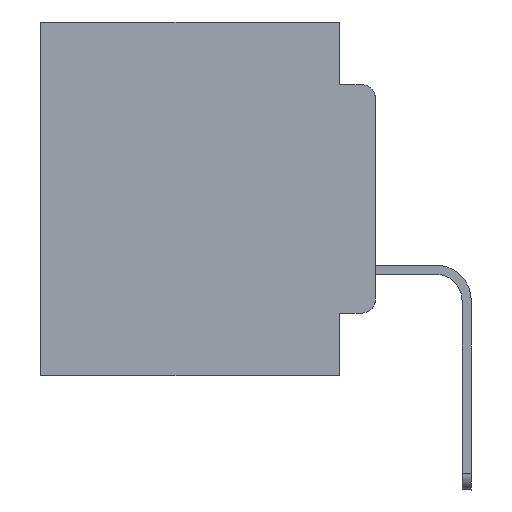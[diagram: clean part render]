
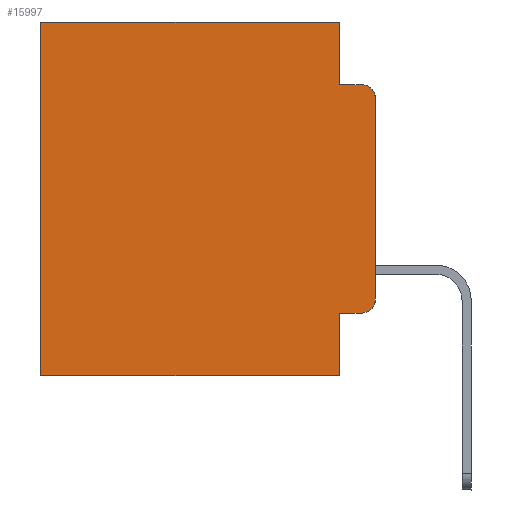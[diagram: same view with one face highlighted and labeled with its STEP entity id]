
A CAD part, left-side view. The second image highlights one B-rep face of the part: STEP entity #15997.
In plain terms, the highlighted planar face has unit normal (-1, 0, 0).
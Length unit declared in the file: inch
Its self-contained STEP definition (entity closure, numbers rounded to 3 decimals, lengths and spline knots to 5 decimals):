
#110 = LINE ( 'NONE', #13488, #19756 ) ;
#147 = DIRECTION ( 'NONE',  ( -1., 0., 0. ) ) ;
#587 = ORIENTED_EDGE ( 'NONE', *, *, #12937, .T. ) ;
#695 = ORIENTED_EDGE ( 'NONE', *, *, #14527, .F. ) ;
#725 = ORIENTED_EDGE ( 'NONE', *, *, #23851, .T. ) ;
#1013 = VERTEX_POINT ( 'NONE', #10838 ) ;
#1475 = LINE ( 'NONE', #11802, #9394 ) ;
#1532 = AXIS2_PLACEMENT_3D ( 'NONE', #22654, #147, #18712 ) ;
#1558 = CARTESIAN_POINT ( 'NONE',  ( 0.298, 0.02, -0.0885 ) ) ;
#2122 = EDGE_CURVE ( 'NONE', #12835, #20879, #1475, .T. ) ;
#2911 = VECTOR ( 'NONE', #20334, 39.37008 ) ;
#2927 = LINE ( 'NONE', #21885, #21627 ) ;
#3465 = CARTESIAN_POINT ( 'NONE',  ( 0.298, 0.051, 0. ) ) ;
#4280 = EDGE_CURVE ( 'NONE', #16893, #9608, #2927, .T. ) ;
#4415 = VECTOR ( 'NONE', #14277, 39.37008 ) ;
#4571 = CARTESIAN_POINT ( 'NONE',  ( 0.298, 0.051, 0. ) ) ;
#4652 = DIRECTION ( 'NONE',  ( 0., 0., -1. ) ) ;
#5561 = CARTESIAN_POINT ( 'NONE',  ( 0.298, 0.02, -0.1085 ) ) ;
#5987 = CARTESIAN_POINT ( 'NONE',  ( 0.298, 0.051, -0.0885 ) ) ;
#6456 = VERTEX_POINT ( 'NONE', #5987 ) ;
#7241 = EDGE_CURVE ( 'NONE', #9608, #1013, #21271, .T. ) ;
#7259 = ORIENTED_EDGE ( 'NONE', *, *, #4280, .F. ) ;
#7428 = DIRECTION ( 'NONE',  ( 0., 0., -1. ) ) ;
#7783 = ORIENTED_EDGE ( 'NONE', *, *, #13882, .T. ) ;
#7812 = DIRECTION ( 'NONE',  ( 0., -1., 0. ) ) ;
#8128 = PLANE ( 'NONE',  #25142 ) ;
#8304 = DIRECTION ( 'NONE',  ( 0., 0., -1. ) ) ;
#8321 = CIRCLE ( 'NONE', #24081, 0.02 ) ;
#9292 = EDGE_CURVE ( 'NONE', #9637, #18678, #14882, .T. ) ;
#9394 = VECTOR ( 'NONE', #15676, 39.37008 ) ;
#9589 = CARTESIAN_POINT ( 'NONE',  ( 0.298, 0.02, -0.4115 ) ) ;
#9608 = VERTEX_POINT ( 'NONE', #25834 ) ;
#9637 = VERTEX_POINT ( 'NONE', #9589 ) ;
#10039 = VECTOR ( 'NONE', #4652, 39.37008 ) ;
#10829 = CARTESIAN_POINT ( 'NONE',  ( 0.298, 0.051, -0.4115 ) ) ;
#10838 = CARTESIAN_POINT ( 'NONE',  ( 0.298, 0.473, -0.5 ) ) ;
#11721 = EDGE_CURVE ( 'NONE', #23690, #18678, #21104, .T. ) ;
#11802 = CARTESIAN_POINT ( 'NONE',  ( 0.298, 0., 0. ) ) ;
#11878 = DIRECTION ( 'NONE',  ( 0., 0., -1. ) ) ;
#12835 = VERTEX_POINT ( 'NONE', #3465 ) ;
#12937 = EDGE_CURVE ( 'NONE', #16893, #9637, #110, .T. ) ;
#13488 = CARTESIAN_POINT ( 'NONE',  ( 0.298, 0.051, -0.4115 ) ) ;
#13882 = EDGE_CURVE ( 'NONE', #20879, #1013, #18330, .T. ) ;
#13915 = ORIENTED_EDGE ( 'NONE', *, *, #9292, .T. ) ;
#14204 = CARTESIAN_POINT ( 'NONE',  ( 0.298, 0.051, -0.0885 ) ) ;
#14277 = DIRECTION ( 'NONE',  ( 0., 1., 0. ) ) ;
#14527 = EDGE_CURVE ( 'NONE', #12835, #6456, #17970, .T. ) ;
#14610 = ORIENTED_EDGE ( 'NONE', *, *, #2122, .T. ) ;
#14773 = ORIENTED_EDGE ( 'NONE', *, *, #7241, .F. ) ;
#14882 = CIRCLE ( 'NONE', #1532, 0.02 ) ;
#15676 = DIRECTION ( 'NONE',  ( 0., 1., 0. ) ) ;
#15867 = LINE ( 'NONE', #14204, #2911 ) ;
#15997 = ADVANCED_FACE ( 'NONE', ( #26174 ), #8128, .F. ) ;
#16629 = VECTOR ( 'NONE', #24293, 39.37008 ) ;
#16640 = VERTEX_POINT ( 'NONE', #1558 ) ;
#16893 = VERTEX_POINT ( 'NONE', #10829 ) ;
#17054 = VECTOR ( 'NONE', #22930, 39.37008 ) ;
#17770 = CARTESIAN_POINT ( 'NONE',  ( 0.298, 0., 0. ) ) ;
#17970 = LINE ( 'NONE', #4571, #10039 ) ;
#18298 = CARTESIAN_POINT ( 'NONE',  ( 0.298, 0., -0.3915 ) ) ;
#18330 = LINE ( 'NONE', #20884, #17054 ) ;
#18678 = VERTEX_POINT ( 'NONE', #18298 ) ;
#18712 = DIRECTION ( 'NONE',  ( 0., 0., -1. ) ) ;
#18906 = CARTESIAN_POINT ( 'NONE',  ( 0.298, 0.473, 0. ) ) ;
#19025 = CARTESIAN_POINT ( 'NONE',  ( 0.298, 0., -0.1085 ) ) ;
#19756 = VECTOR ( 'NONE', #7812, 39.37008 ) ;
#20334 = DIRECTION ( 'NONE',  ( 0., -1., 0. ) ) ;
#20879 = VERTEX_POINT ( 'NONE', #18906 ) ;
#20884 = CARTESIAN_POINT ( 'NONE',  ( 0.298, 0.473, 0. ) ) ;
#21104 = LINE ( 'NONE', #17770, #16629 ) ;
#21271 = LINE ( 'NONE', #24770, #4415 ) ;
#21467 = EDGE_LOOP ( 'NONE', ( #24245, #725, #22363, #695, #14610, #7783, #14773, #7259, #587, #13915 ) ) ;
#21627 = VECTOR ( 'NONE', #11878, 39.37008 ) ;
#21885 = CARTESIAN_POINT ( 'NONE',  ( 0.298, 0.051, 0. ) ) ;
#22322 = CARTESIAN_POINT ( 'NONE',  ( 0.298, 0., 0. ) ) ;
#22363 = ORIENTED_EDGE ( 'NONE', *, *, #24744, .F. ) ;
#22654 = CARTESIAN_POINT ( 'NONE',  ( 0.298, 0.02, -0.3915 ) ) ;
#22930 = DIRECTION ( 'NONE',  ( 0., 0., -1. ) ) ;
#23652 = DIRECTION ( 'NONE',  ( -1., 0., 0. ) ) ;
#23690 = VERTEX_POINT ( 'NONE', #19025 ) ;
#23851 = EDGE_CURVE ( 'NONE', #23690, #16640, #8321, .T. ) ;
#24081 = AXIS2_PLACEMENT_3D ( 'NONE', #5561, #23652, #7428 ) ;
#24245 = ORIENTED_EDGE ( 'NONE', *, *, #11721, .F. ) ;
#24293 = DIRECTION ( 'NONE',  ( 0., 0., -1. ) ) ;
#24475 = DIRECTION ( 'NONE',  ( 1., 0., 0. ) ) ;
#24744 = EDGE_CURVE ( 'NONE', #6456, #16640, #15867, .T. ) ;
#24770 = CARTESIAN_POINT ( 'NONE',  ( 0.298, 0., -0.5 ) ) ;
#25142 = AXIS2_PLACEMENT_3D ( 'NONE', #22322, #24475, #8304 ) ;
#25834 = CARTESIAN_POINT ( 'NONE',  ( 0.298, 0.051, -0.5 ) ) ;
#26174 = FACE_OUTER_BOUND ( 'NONE', #21467, .T. ) ;
